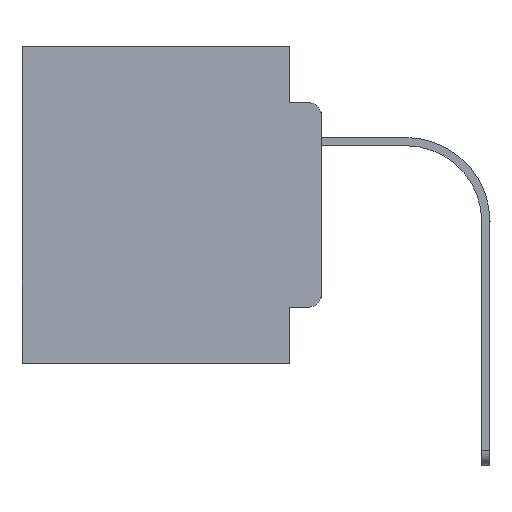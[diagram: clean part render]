
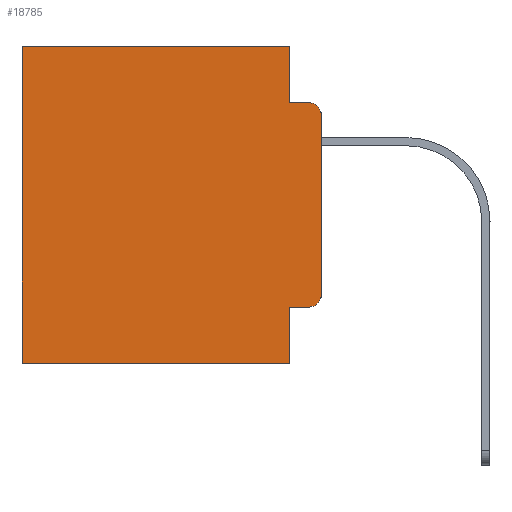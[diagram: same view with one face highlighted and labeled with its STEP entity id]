
A CAD part, left-side view. The second image highlights one B-rep face of the part: STEP entity #18785.
In plain terms, the highlighted planar face has unit normal (-1, 0, 0).
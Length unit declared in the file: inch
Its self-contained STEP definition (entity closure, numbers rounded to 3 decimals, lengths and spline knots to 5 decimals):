
#1570 = CARTESIAN_POINT ( 'NONE',  ( 0.298, 0., 0. ) ) ;
#1614 = LINE ( 'NONE', #17163, #10396 ) ;
#1791 = CARTESIAN_POINT ( 'NONE',  ( 0.298, 0.051, -0.0885 ) ) ;
#2252 = CARTESIAN_POINT ( 'NONE',  ( 0.298, 0., -0.3915 ) ) ;
#2564 = EDGE_CURVE ( 'NONE', #22954, #5675, #17360, .T. ) ;
#2737 = VECTOR ( 'NONE', #8485, 39.37008 ) ;
#3174 = CARTESIAN_POINT ( 'NONE',  ( 0.298, 0.051, -0.4115 ) ) ;
#3479 = ORIENTED_EDGE ( 'NONE', *, *, #28318, .F. ) ;
#3576 = CIRCLE ( 'NONE', #10939, 0.02 ) ;
#3646 = ORIENTED_EDGE ( 'NONE', *, *, #22141, .T. ) ;
#3744 = VECTOR ( 'NONE', #20340, 39.37008 ) ;
#3929 = CARTESIAN_POINT ( 'NONE',  ( 0.298, 0.02, -0.0885 ) ) ;
#4583 = EDGE_CURVE ( 'NONE', #13478, #16731, #7752, .T. ) ;
#4824 = VECTOR ( 'NONE', #9426, 39.37008 ) ;
#5675 = VERTEX_POINT ( 'NONE', #7310 ) ;
#5768 = PLANE ( 'NONE',  #19617 ) ;
#5982 = VERTEX_POINT ( 'NONE', #2252 ) ;
#6590 = CARTESIAN_POINT ( 'NONE',  ( 0.298, 0.051, 0. ) ) ;
#6707 = CARTESIAN_POINT ( 'NONE',  ( 0.298, 0.02, -0.3915 ) ) ;
#7102 = VERTEX_POINT ( 'NONE', #16680 ) ;
#7269 = LINE ( 'NONE', #9300, #20264 ) ;
#7310 = CARTESIAN_POINT ( 'NONE',  ( 0.298, 0.051, -0.5 ) ) ;
#7601 = DIRECTION ( 'NONE',  ( 0., 0., -1. ) ) ;
#7752 = LINE ( 'NONE', #27787, #26242 ) ;
#8086 = DIRECTION ( 'NONE',  ( 1., 0., 0. ) ) ;
#8349 = LINE ( 'NONE', #15512, #20846 ) ;
#8485 = DIRECTION ( 'NONE',  ( 0., 1., 0. ) ) ;
#9236 = CARTESIAN_POINT ( 'NONE',  ( 0.298, 0., -0.5 ) ) ;
#9300 = CARTESIAN_POINT ( 'NONE',  ( 0.298, 0.051, -0.4115 ) ) ;
#9426 = DIRECTION ( 'NONE',  ( 0., 0., -1. ) ) ;
#9736 = DIRECTION ( 'NONE',  ( 0., -1., 0. ) ) ;
#9903 = ORIENTED_EDGE ( 'NONE', *, *, #2564, .F. ) ;
#10396 = VECTOR ( 'NONE', #25983, 39.37008 ) ;
#10435 = ORIENTED_EDGE ( 'NONE', *, *, #13900, .T. ) ;
#10939 = AXIS2_PLACEMENT_3D ( 'NONE', #27343, #16667, #7601 ) ;
#11734 = EDGE_LOOP ( 'NONE', ( #3479, #3646, #27361, #22140, #13959, #27504, #16351, #9903, #23934, #10435 ) ) ;
#11813 = CARTESIAN_POINT ( 'NONE',  ( 0.298, 0., -0.1085 ) ) ;
#12119 = VERTEX_POINT ( 'NONE', #6590 ) ;
#13231 = EDGE_CURVE ( 'NONE', #12119, #13478, #16697, .T. ) ;
#13340 = DIRECTION ( 'NONE',  ( -1., 0., 0. ) ) ;
#13478 = VERTEX_POINT ( 'NONE', #24484 ) ;
#13900 = EDGE_CURVE ( 'NONE', #7102, #5982, #26265, .T. ) ;
#13959 = ORIENTED_EDGE ( 'NONE', *, *, #13231, .T. ) ;
#14113 = DIRECTION ( 'NONE',  ( 0., -1., 0. ) ) ;
#14410 = CARTESIAN_POINT ( 'NONE',  ( 0.298, 0., 0. ) ) ;
#15512 = CARTESIAN_POINT ( 'NONE',  ( 0.298, 0., 0. ) ) ;
#15960 = VERTEX_POINT ( 'NONE', #3929 ) ;
#16030 = CARTESIAN_POINT ( 'NONE',  ( 0.298, 0.051, 0. ) ) ;
#16351 = ORIENTED_EDGE ( 'NONE', *, *, #26666, .F. ) ;
#16667 = DIRECTION ( 'NONE',  ( -1., 0., 0. ) ) ;
#16680 = CARTESIAN_POINT ( 'NONE',  ( 0.298, 0.02, -0.4115 ) ) ;
#16697 = LINE ( 'NONE', #1570, #2737 ) ;
#16731 = VERTEX_POINT ( 'NONE', #17204 ) ;
#17078 = VECTOR ( 'NONE', #14113, 39.37008 ) ;
#17163 = CARTESIAN_POINT ( 'NONE',  ( 0.298, 0.051, 0. ) ) ;
#17204 = CARTESIAN_POINT ( 'NONE',  ( 0.298, 0.473, -0.5 ) ) ;
#17360 = LINE ( 'NONE', #16030, #4824 ) ;
#17681 = DIRECTION ( 'NONE',  ( 0., 0., -1. ) ) ;
#18593 = CARTESIAN_POINT ( 'NONE',  ( 0.298, 0.051, -0.0885 ) ) ;
#18785 = ADVANCED_FACE ( 'NONE', ( #27398 ), #5768, .F. ) ;
#19552 = DIRECTION ( 'NONE',  ( 0., 0., -1. ) ) ;
#19617 = AXIS2_PLACEMENT_3D ( 'NONE', #14410, #8086, #27694 ) ;
#20062 = LINE ( 'NONE', #9236, #3744 ) ;
#20211 = EDGE_CURVE ( 'NONE', #12119, #27175, #1614, .T. ) ;
#20264 = VECTOR ( 'NONE', #9736, 39.37008 ) ;
#20340 = DIRECTION ( 'NONE',  ( 0., 1., 0. ) ) ;
#20846 = VECTOR ( 'NONE', #17681, 39.37008 ) ;
#21320 = DIRECTION ( 'NONE',  ( 0., 0., -1. ) ) ;
#22134 = AXIS2_PLACEMENT_3D ( 'NONE', #6707, #13340, #19552 ) ;
#22140 = ORIENTED_EDGE ( 'NONE', *, *, #20211, .F. ) ;
#22141 = EDGE_CURVE ( 'NONE', #28103, #15960, #3576, .T. ) ;
#22954 = VERTEX_POINT ( 'NONE', #3174 ) ;
#23934 = ORIENTED_EDGE ( 'NONE', *, *, #24463, .T. ) ;
#24463 = EDGE_CURVE ( 'NONE', #22954, #7102, #7269, .T. ) ;
#24484 = CARTESIAN_POINT ( 'NONE',  ( 0.298, 0.473, 0. ) ) ;
#25678 = LINE ( 'NONE', #18593, #17078 ) ;
#25983 = DIRECTION ( 'NONE',  ( 0., 0., -1. ) ) ;
#26242 = VECTOR ( 'NONE', #21320, 39.37008 ) ;
#26265 = CIRCLE ( 'NONE', #22134, 0.02 ) ;
#26666 = EDGE_CURVE ( 'NONE', #5675, #16731, #20062, .T. ) ;
#26784 = EDGE_CURVE ( 'NONE', #27175, #15960, #25678, .T. ) ;
#27175 = VERTEX_POINT ( 'NONE', #1791 ) ;
#27343 = CARTESIAN_POINT ( 'NONE',  ( 0.298, 0.02, -0.1085 ) ) ;
#27361 = ORIENTED_EDGE ( 'NONE', *, *, #26784, .F. ) ;
#27398 = FACE_OUTER_BOUND ( 'NONE', #11734, .T. ) ;
#27504 = ORIENTED_EDGE ( 'NONE', *, *, #4583, .T. ) ;
#27694 = DIRECTION ( 'NONE',  ( 0., 0., -1. ) ) ;
#27787 = CARTESIAN_POINT ( 'NONE',  ( 0.298, 0.473, 0. ) ) ;
#28103 = VERTEX_POINT ( 'NONE', #11813 ) ;
#28318 = EDGE_CURVE ( 'NONE', #28103, #5982, #8349, .T. ) ;
